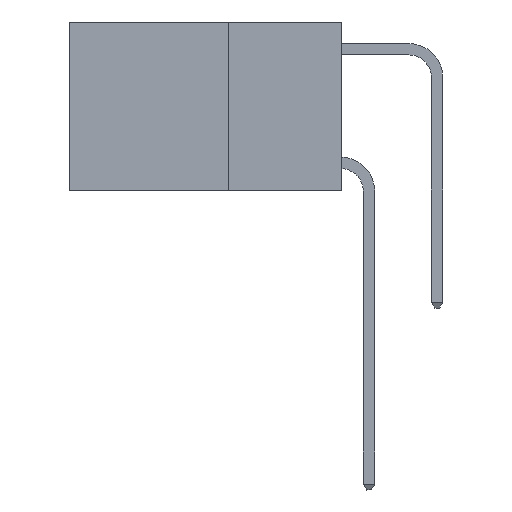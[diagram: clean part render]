
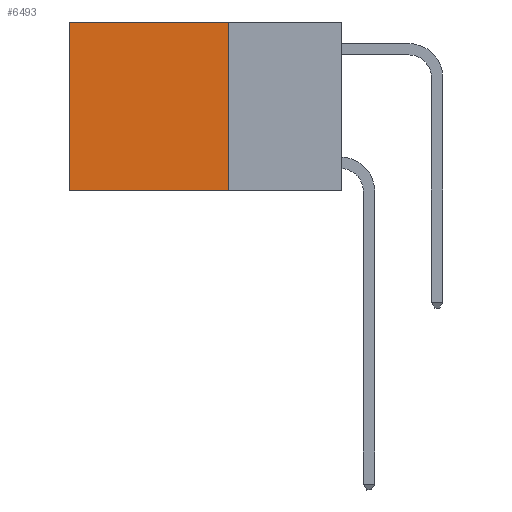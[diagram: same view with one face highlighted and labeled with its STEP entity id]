
A CAD part, left-side view. The second image highlights one B-rep face of the part: STEP entity #6493.
In plain terms, the highlighted planar face has unit normal (-1, 0, 0).
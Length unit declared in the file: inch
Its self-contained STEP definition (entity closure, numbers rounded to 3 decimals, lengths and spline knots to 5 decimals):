
#261 = CARTESIAN_POINT ( 'NONE',  ( 0.2625, 0.25, -0.37 ) ) ;
#1530 = VECTOR ( 'NONE', #2784, 39.37008 ) ;
#1535 = PLANE ( 'NONE',  #12762 ) ;
#2203 = VECTOR ( 'NONE', #6794, 39.37008 ) ;
#2784 = DIRECTION ( 'NONE',  ( 0., 1., 0. ) ) ;
#3017 = DIRECTION ( 'NONE',  ( 0., 0., -1. ) ) ;
#3182 = VERTEX_POINT ( 'NONE', #261 ) ;
#3197 = DIRECTION ( 'NONE',  ( 0., 0., -1. ) ) ;
#3508 = FACE_OUTER_BOUND ( 'NONE', #5525, .T. ) ;
#3652 = CARTESIAN_POINT ( 'NONE',  ( 0.2625, 0.25, 0. ) ) ;
#4370 = CARTESIAN_POINT ( 'NONE',  ( 0.2625, 0.6, 0. ) ) ;
#4506 = VECTOR ( 'NONE', #3197, 39.37008 ) ;
#4710 = DIRECTION ( 'NONE',  ( 0., 0., -1. ) ) ;
#4919 = EDGE_CURVE ( 'NONE', #11956, #12408, #7895, .T. ) ;
#4930 = VECTOR ( 'NONE', #3017, 39.37008 ) ;
#5525 = EDGE_LOOP ( 'NONE', ( #8347, #8178, #9295, #7406 ) ) ;
#6220 = CARTESIAN_POINT ( 'NONE',  ( 0.2625, 0.6, -0.37 ) ) ;
#6493 = ADVANCED_FACE ( 'NONE', ( #3508 ), #1535, .F. ) ;
#6605 = EDGE_CURVE ( 'NONE', #3182, #12408, #12319, .T. ) ;
#6794 = DIRECTION ( 'NONE',  ( 0., 1., 0. ) ) ;
#6835 = CARTESIAN_POINT ( 'NONE',  ( 0.2625, 0.25, 0. ) ) ;
#7176 = LINE ( 'NONE', #7241, #4506 ) ;
#7241 = CARTESIAN_POINT ( 'NONE',  ( 0.2625, 0.25, 0. ) ) ;
#7406 = ORIENTED_EDGE ( 'NONE', *, *, #12164, .T. ) ;
#7844 = CARTESIAN_POINT ( 'NONE',  ( 0.2625, 0.25, -0.37 ) ) ;
#7895 = LINE ( 'NONE', #13023, #4930 ) ;
#8178 = ORIENTED_EDGE ( 'NONE', *, *, #6605, .F. ) ;
#8347 = ORIENTED_EDGE ( 'NONE', *, *, #4919, .T. ) ;
#8936 = VERTEX_POINT ( 'NONE', #9683 ) ;
#9295 = ORIENTED_EDGE ( 'NONE', *, *, #13020, .F. ) ;
#9683 = CARTESIAN_POINT ( 'NONE',  ( 0.2625, 0.25, 0. ) ) ;
#10735 = DIRECTION ( 'NONE',  ( 1., 0., 0. ) ) ;
#11956 = VERTEX_POINT ( 'NONE', #4370 ) ;
#12164 = EDGE_CURVE ( 'NONE', #8936, #11956, #12617, .T. ) ;
#12319 = LINE ( 'NONE', #7844, #1530 ) ;
#12408 = VERTEX_POINT ( 'NONE', #6220 ) ;
#12617 = LINE ( 'NONE', #6835, #2203 ) ;
#12762 = AXIS2_PLACEMENT_3D ( 'NONE', #3652, #10735, #4710 ) ;
#13020 = EDGE_CURVE ( 'NONE', #8936, #3182, #7176, .T. ) ;
#13023 = CARTESIAN_POINT ( 'NONE',  ( 0.2625, 0.6, 0. ) ) ;
